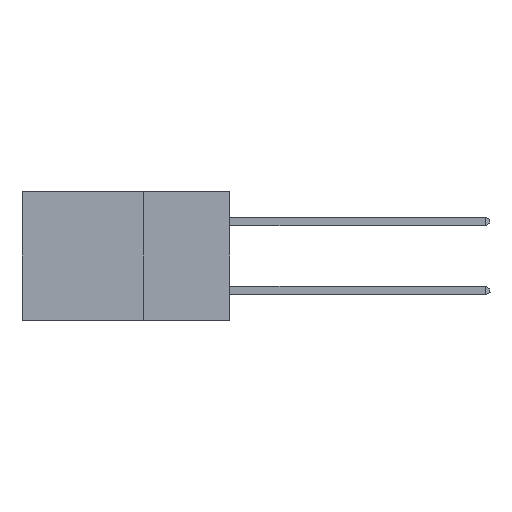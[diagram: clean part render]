
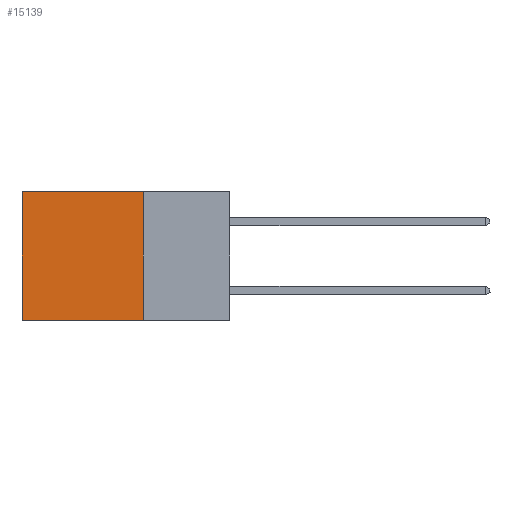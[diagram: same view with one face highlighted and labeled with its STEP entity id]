
A CAD part, left-side view. The second image highlights one B-rep face of the part: STEP entity #15139.
In plain terms, the highlighted planar face has unit normal (-1, 0, 0).
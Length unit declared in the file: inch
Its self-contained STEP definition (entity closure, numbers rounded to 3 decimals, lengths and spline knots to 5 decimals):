
#26 = EDGE_LOOP ( 'NONE', ( #8815, #11404, #1242, #6625 ) ) ;
#1242 = ORIENTED_EDGE ( 'NONE', *, *, #8540, .F. ) ;
#1403 = VECTOR ( 'NONE', #11759, 39.37008 ) ;
#1486 = VERTEX_POINT ( 'NONE', #12818 ) ;
#1728 = PLANE ( 'NONE',  #9526 ) ;
#2127 = EDGE_CURVE ( 'NONE', #5021, #8513, #7970, .T. ) ;
#2508 = CARTESIAN_POINT ( 'NONE',  ( 0.298, 0.6, 0. ) ) ;
#3205 = CARTESIAN_POINT ( 'NONE',  ( 0.298, 0.25, -0.37 ) ) ;
#3215 = CARTESIAN_POINT ( 'NONE',  ( 0.298, 0.25, -0.37 ) ) ;
#4830 = EDGE_CURVE ( 'NONE', #12861, #8513, #13672, .T. ) ;
#5021 = VERTEX_POINT ( 'NONE', #3205 ) ;
#5518 = DIRECTION ( 'NONE',  ( 0., 0., -1. ) ) ;
#5535 = EDGE_CURVE ( 'NONE', #1486, #12861, #9335, .T. ) ;
#6625 = ORIENTED_EDGE ( 'NONE', *, *, #5535, .T. ) ;
#6642 = DIRECTION ( 'NONE',  ( 0., 0., -1. ) ) ;
#7314 = VECTOR ( 'NONE', #10885, 39.37008 ) ;
#7970 = LINE ( 'NONE', #3215, #1403 ) ;
#8513 = VERTEX_POINT ( 'NONE', #12417 ) ;
#8540 = EDGE_CURVE ( 'NONE', #1486, #5021, #11621, .T. ) ;
#8815 = ORIENTED_EDGE ( 'NONE', *, *, #4830, .T. ) ;
#9175 = CARTESIAN_POINT ( 'NONE',  ( 0.298, 0.25, 0. ) ) ;
#9335 = LINE ( 'NONE', #9175, #13082 ) ;
#9526 = AXIS2_PLACEMENT_3D ( 'NONE', #13798, #10092, #6642 ) ;
#10092 = DIRECTION ( 'NONE',  ( 1., 0., 0. ) ) ;
#10690 = VECTOR ( 'NONE', #5518, 39.37008 ) ;
#10885 = DIRECTION ( 'NONE',  ( 0., 0., -1. ) ) ;
#11373 = CARTESIAN_POINT ( 'NONE',  ( 0.298, 0.25, 0. ) ) ;
#11404 = ORIENTED_EDGE ( 'NONE', *, *, #2127, .F. ) ;
#11621 = LINE ( 'NONE', #11373, #10690 ) ;
#11759 = DIRECTION ( 'NONE',  ( 0., 1., 0. ) ) ;
#12417 = CARTESIAN_POINT ( 'NONE',  ( 0.298, 0.6, -0.37 ) ) ;
#12818 = CARTESIAN_POINT ( 'NONE',  ( 0.298, 0.25, 0. ) ) ;
#12861 = VERTEX_POINT ( 'NONE', #14553 ) ;
#12892 = DIRECTION ( 'NONE',  ( 0., 1., 0. ) ) ;
#13082 = VECTOR ( 'NONE', #12892, 39.37008 ) ;
#13672 = LINE ( 'NONE', #2508, #7314 ) ;
#13798 = CARTESIAN_POINT ( 'NONE',  ( 0.298, 0.25, 0. ) ) ;
#14229 = FACE_OUTER_BOUND ( 'NONE', #26, .T. ) ;
#14553 = CARTESIAN_POINT ( 'NONE',  ( 0.298, 0.6, 0. ) ) ;
#15139 = ADVANCED_FACE ( 'NONE', ( #14229 ), #1728, .F. ) ;
